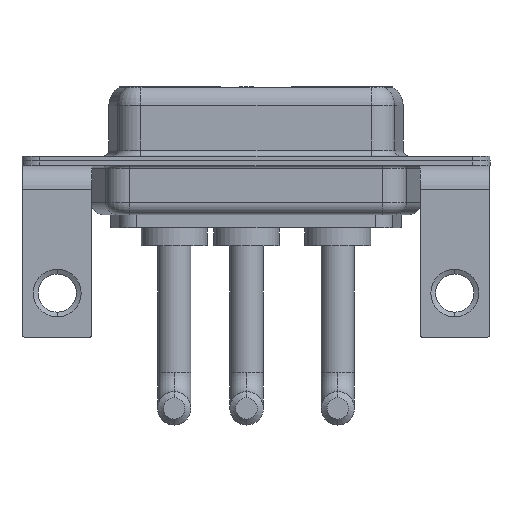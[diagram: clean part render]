
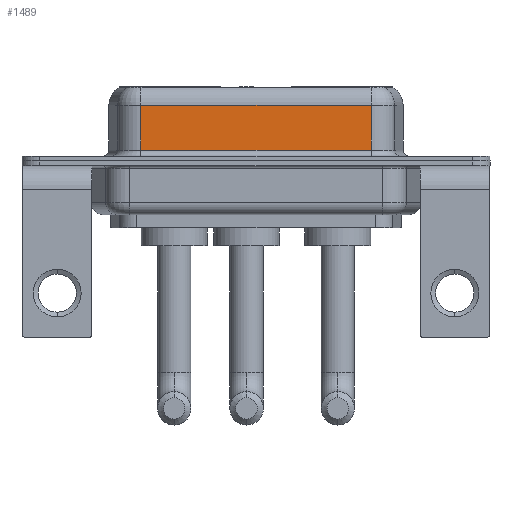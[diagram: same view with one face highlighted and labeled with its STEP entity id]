
A CAD part, front view. The second image highlights one B-rep face of the part: STEP entity #1489.
In plain terms, the highlighted planar face has unit normal (0, -1, 0).
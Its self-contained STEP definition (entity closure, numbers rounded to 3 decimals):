
#587 = ORIENTED_EDGE ( 'NONE', *, *, #3796, .T. ) ;
#598 = EDGE_CURVE ( 'NONE', #13550, #9768, #3916, .T. ) ;
#963 = DIRECTION ( 'NONE',  ( 0., 0., 1. ) ) ;
#1036 = EDGE_LOOP ( 'NONE', ( #6452, #7921, #12863, #587 ) ) ;
#1231 = VERTEX_POINT ( 'NONE', #11929 ) ;
#1489 = ADVANCED_FACE ( 'NONE', ( #10095 ), #11040, .F. ) ;
#2138 = CARTESIAN_POINT ( 'NONE',  ( 26.287, -3.95, 6.4 ) ) ;
#2380 = CARTESIAN_POINT ( 'NONE',  ( 26.287, -3.95, 0.9 ) ) ;
#2452 = DIRECTION ( 'NONE',  ( -1., 0., 0. ) ) ;
#2520 = LINE ( 'NONE', #5691, #13411 ) ;
#3336 = VECTOR ( 'NONE', #3708, 1000. ) ;
#3708 = DIRECTION ( 'NONE',  ( 0., 0., -1. ) ) ;
#3796 = EDGE_CURVE ( 'NONE', #1231, #9768, #10401, .T. ) ;
#3916 = LINE ( 'NONE', #7089, #3336 ) ;
#4289 = VECTOR ( 'NONE', #5906, 1000. ) ;
#5691 = CARTESIAN_POINT ( 'NONE',  ( 26.287, -3.95, 4.65 ) ) ;
#5826 = VECTOR ( 'NONE', #10261, 1000. ) ;
#5906 = DIRECTION ( 'NONE',  ( 1., 0., 0. ) ) ;
#6452 = ORIENTED_EDGE ( 'NONE', *, *, #598, .F. ) ;
#7089 = CARTESIAN_POINT ( 'NONE',  ( 26.287, -3.95, 6.4 ) ) ;
#7700 = CARTESIAN_POINT ( 'NONE',  ( 7.013, -3.95, 4.65 ) ) ;
#7921 = ORIENTED_EDGE ( 'NONE', *, *, #12460, .T. ) ;
#8567 = CARTESIAN_POINT ( 'NONE',  ( 26.287, -3.95, 4.65 ) ) ;
#9768 = VERTEX_POINT ( 'NONE', #14249 ) ;
#10063 = EDGE_CURVE ( 'NONE', #10527, #1231, #12958, .T. ) ;
#10095 = FACE_OUTER_BOUND ( 'NONE', #1036, .T. ) ;
#10261 = DIRECTION ( 'NONE',  ( 0., 0., -1. ) ) ;
#10401 = LINE ( 'NONE', #2380, #4289 ) ;
#10527 = VERTEX_POINT ( 'NONE', #7700 ) ;
#11040 = PLANE ( 'NONE',  #13322 ) ;
#11187 = DIRECTION ( 'NONE',  ( 0., 1., 0. ) ) ;
#11849 = CARTESIAN_POINT ( 'NONE',  ( 7.013, -3.95, 6.4 ) ) ;
#11929 = CARTESIAN_POINT ( 'NONE',  ( 7.013, -3.95, 0.9 ) ) ;
#12460 = EDGE_CURVE ( 'NONE', #13550, #10527, #2520, .T. ) ;
#12863 = ORIENTED_EDGE ( 'NONE', *, *, #10063, .T. ) ;
#12958 = LINE ( 'NONE', #11849, #5826 ) ;
#13322 = AXIS2_PLACEMENT_3D ( 'NONE', #2138, #11187, #963 ) ;
#13411 = VECTOR ( 'NONE', #2452, 1000. ) ;
#13550 = VERTEX_POINT ( 'NONE', #8567 ) ;
#14249 = CARTESIAN_POINT ( 'NONE',  ( 26.287, -3.95, 0.9 ) ) ;
